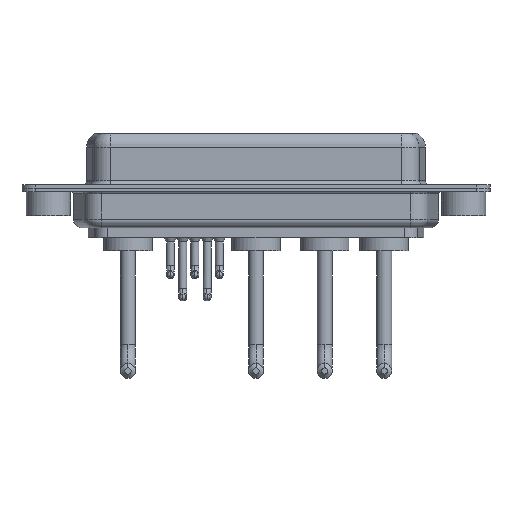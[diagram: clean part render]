
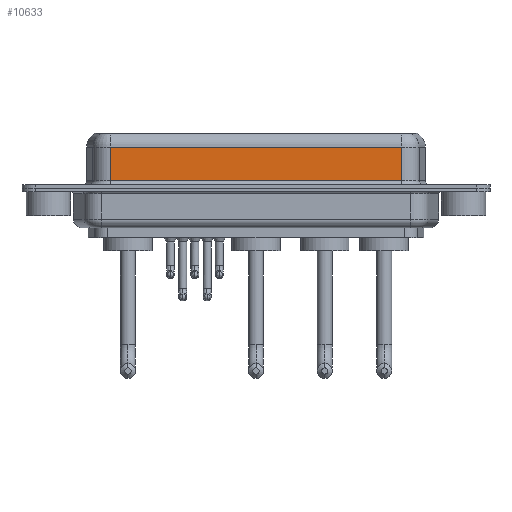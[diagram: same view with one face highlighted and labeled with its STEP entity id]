
A CAD part, front view. The second image highlights one B-rep face of the part: STEP entity #10633.
In plain terms, the highlighted planar face has unit normal (0, -1, 0).
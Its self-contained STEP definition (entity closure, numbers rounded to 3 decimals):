
#548 = EDGE_LOOP ( 'NONE', ( #10483, #5246, #3210, #8123 ) ) ;
#657 = CARTESIAN_POINT ( 'NONE',  ( 7.013, -3.95, 6.4 ) ) ;
#1864 = CARTESIAN_POINT ( 'NONE',  ( 40.037, -3.95, 6.4 ) ) ;
#2140 = LINE ( 'NONE', #5012, #9078 ) ;
#2778 = LINE ( 'NONE', #10361, #14356 ) ;
#3055 = EDGE_CURVE ( 'NONE', #10597, #11809, #2778, .T. ) ;
#3210 = ORIENTED_EDGE ( 'NONE', *, *, #6703, .T. ) ;
#5012 = CARTESIAN_POINT ( 'NONE',  ( 40.037, -3.95, 4.65 ) ) ;
#5246 = ORIENTED_EDGE ( 'NONE', *, *, #6755, .T. ) ;
#5283 = DIRECTION ( 'NONE',  ( 1., 0., 0. ) ) ;
#5757 = CARTESIAN_POINT ( 'NONE',  ( 7.013, -3.95, 4.65 ) ) ;
#5868 = CARTESIAN_POINT ( 'NONE',  ( 7.013, -3.95, 0.9 ) ) ;
#6703 = EDGE_CURVE ( 'NONE', #11662, #16671, #12616, .T. ) ;
#6755 = EDGE_CURVE ( 'NONE', #10597, #11662, #2140, .T. ) ;
#7235 = CARTESIAN_POINT ( 'NONE',  ( 40.037, -3.95, 0.9 ) ) ;
#8123 = ORIENTED_EDGE ( 'NONE', *, *, #12255, .T. ) ;
#8637 = VECTOR ( 'NONE', #5283, 1000. ) ;
#9078 = VECTOR ( 'NONE', #12700, 1000. ) ;
#9731 = DIRECTION ( 'NONE',  ( 0., 1., 0. ) ) ;
#10361 = CARTESIAN_POINT ( 'NONE',  ( 40.037, -3.95, 6.4 ) ) ;
#10483 = ORIENTED_EDGE ( 'NONE', *, *, #3055, .F. ) ;
#10597 = VERTEX_POINT ( 'NONE', #17033 ) ;
#10607 = PLANE ( 'NONE',  #14757 ) ;
#10633 = ADVANCED_FACE ( 'NONE', ( #11588 ), #10607, .F. ) ;
#10938 = LINE ( 'NONE', #13480, #8637 ) ;
#11588 = FACE_OUTER_BOUND ( 'NONE', #548, .T. ) ;
#11662 = VERTEX_POINT ( 'NONE', #5757 ) ;
#11809 = VERTEX_POINT ( 'NONE', #7235 ) ;
#11930 = DIRECTION ( 'NONE',  ( 0., 0., -1. ) ) ;
#12255 = EDGE_CURVE ( 'NONE', #16671, #11809, #10938, .T. ) ;
#12616 = LINE ( 'NONE', #657, #16628 ) ;
#12700 = DIRECTION ( 'NONE',  ( -1., 0., 0. ) ) ;
#13480 = CARTESIAN_POINT ( 'NONE',  ( 40.037, -3.95, 0.9 ) ) ;
#14356 = VECTOR ( 'NONE', #11930, 1000. ) ;
#14654 = DIRECTION ( 'NONE',  ( 0., 0., 1. ) ) ;
#14757 = AXIS2_PLACEMENT_3D ( 'NONE', #1864, #9731, #14654 ) ;
#16087 = DIRECTION ( 'NONE',  ( 0., 0., -1. ) ) ;
#16628 = VECTOR ( 'NONE', #16087, 1000. ) ;
#16671 = VERTEX_POINT ( 'NONE', #5868 ) ;
#17033 = CARTESIAN_POINT ( 'NONE',  ( 40.037, -3.95, 4.65 ) ) ;
